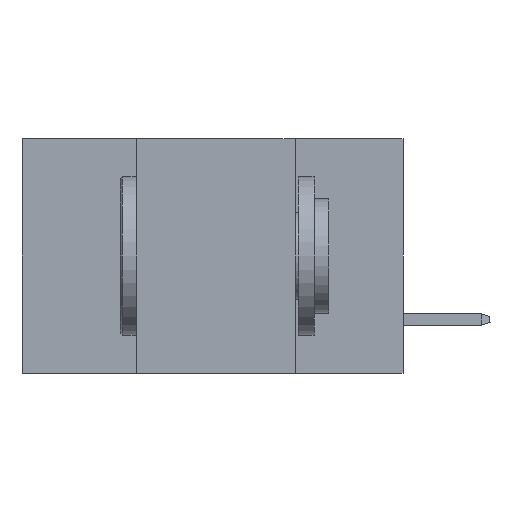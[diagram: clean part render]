
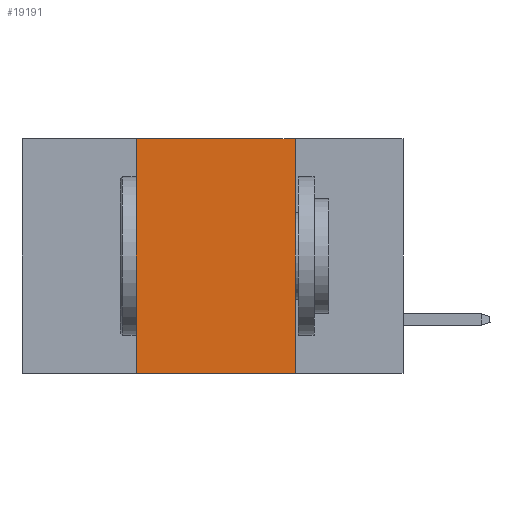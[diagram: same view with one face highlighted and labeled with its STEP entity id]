
A CAD part, left-side view. The second image highlights one B-rep face of the part: STEP entity #19191.
In plain terms, the highlighted planar face has unit normal (-1, 0, 0).
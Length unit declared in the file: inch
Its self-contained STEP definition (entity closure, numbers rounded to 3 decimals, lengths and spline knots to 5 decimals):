
#189 = CARTESIAN_POINT ( 'NONE',  ( 0., 0.6, -0.37 ) ) ;
#240 = LINE ( 'NONE', #4494, #12318 ) ;
#295 = LINE ( 'NONE', #14006, #25238 ) ;
#865 = VECTOR ( 'NONE', #20259, 39.37008 ) ;
#1875 = AXIS2_PLACEMENT_3D ( 'NONE', #26075, #11855, #20068 ) ;
#2503 = ORIENTED_EDGE ( 'NONE', *, *, #22824, .F. ) ;
#2968 = CARTESIAN_POINT ( 'NONE',  ( 0., 0.42, -0.37 ) ) ;
#3012 = EDGE_CURVE ( 'NONE', #7368, #17656, #295, .T. ) ;
#4157 = DIRECTION ( 'NONE',  ( 0., -1., 0. ) ) ;
#4494 = CARTESIAN_POINT ( 'NONE',  ( 0., 0.42, 0. ) ) ;
#5717 = FACE_OUTER_BOUND ( 'NONE', #12927, .T. ) ;
#5836 = PLANE ( 'NONE',  #1875 ) ;
#6488 = DIRECTION ( 'NONE',  ( 0., 0., 1. ) ) ;
#7368 = VERTEX_POINT ( 'NONE', #14173 ) ;
#7776 = VECTOR ( 'NONE', #17509, 39.37008 ) ;
#9241 = EDGE_CURVE ( 'NONE', #23411, #20020, #16131, .T. ) ;
#11288 = CARTESIAN_POINT ( 'NONE',  ( 0., 0.17, 0. ) ) ;
#11855 = DIRECTION ( 'NONE',  ( 1., 0., 0. ) ) ;
#11935 = CARTESIAN_POINT ( 'NONE',  ( 0., 0.17, -0.37 ) ) ;
#12318 = VECTOR ( 'NONE', #6488, 39.37008 ) ;
#12927 = EDGE_LOOP ( 'NONE', ( #17381, #20037, #2503, #15263 ) ) ;
#14006 = CARTESIAN_POINT ( 'NONE',  ( 0., 0.6, 0. ) ) ;
#14173 = CARTESIAN_POINT ( 'NONE',  ( 0., 0.42, 0. ) ) ;
#15263 = ORIENTED_EDGE ( 'NONE', *, *, #9241, .T. ) ;
#16131 = LINE ( 'NONE', #189, #865 ) ;
#17064 = CARTESIAN_POINT ( 'NONE',  ( 0., 0.17, 0. ) ) ;
#17381 = ORIENTED_EDGE ( 'NONE', *, *, #18052, .F. ) ;
#17509 = DIRECTION ( 'NONE',  ( 0., 0., -1. ) ) ;
#17656 = VERTEX_POINT ( 'NONE', #17064 ) ;
#18052 = EDGE_CURVE ( 'NONE', #17656, #20020, #21761, .T. ) ;
#19191 = ADVANCED_FACE ( 'NONE', ( #5717 ), #5836, .F. ) ;
#20020 = VERTEX_POINT ( 'NONE', #11935 ) ;
#20037 = ORIENTED_EDGE ( 'NONE', *, *, #3012, .F. ) ;
#20068 = DIRECTION ( 'NONE',  ( 0., 0., -1. ) ) ;
#20259 = DIRECTION ( 'NONE',  ( 0., -1., 0. ) ) ;
#21761 = LINE ( 'NONE', #11288, #7776 ) ;
#22824 = EDGE_CURVE ( 'NONE', #23411, #7368, #240, .T. ) ;
#23411 = VERTEX_POINT ( 'NONE', #2968 ) ;
#25238 = VECTOR ( 'NONE', #4157, 39.37008 ) ;
#26075 = CARTESIAN_POINT ( 'NONE',  ( 0., 0.6, 0. ) ) ;
